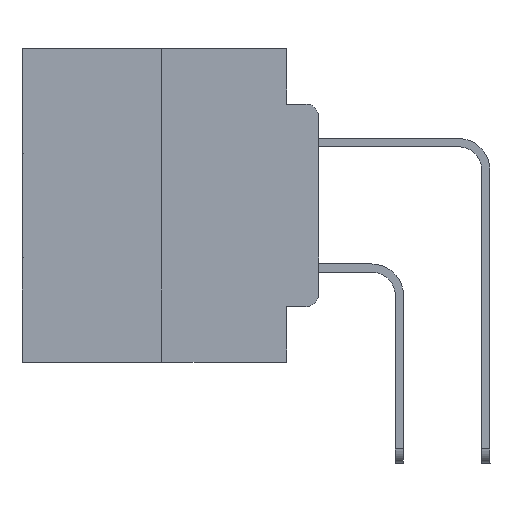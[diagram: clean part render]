
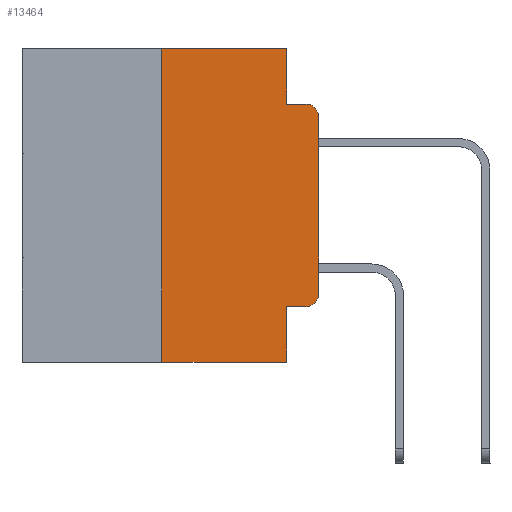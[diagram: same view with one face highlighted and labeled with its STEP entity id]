
A CAD part, left-side view. The second image highlights one B-rep face of the part: STEP entity #13464.
In plain terms, the highlighted planar face has unit normal (-1, 0, 0).
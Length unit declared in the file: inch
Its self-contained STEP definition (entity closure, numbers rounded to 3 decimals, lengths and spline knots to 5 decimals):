
#672 = LINE ( 'NONE', #13309, #23702 ) ;
#1261 = EDGE_CURVE ( 'NONE', #27705, #19291, #21496, .T. ) ;
#1399 = VERTEX_POINT ( 'NONE', #1431 ) ;
#1431 = CARTESIAN_POINT ( 'NONE',  ( 0., 0.25, 0. ) ) ;
#1716 = DIRECTION ( 'NONE',  ( 0., -1., 0. ) ) ;
#2072 = LINE ( 'NONE', #10075, #24971 ) ;
#3303 = CARTESIAN_POINT ( 'NONE',  ( 0., 0.051, -0.0885 ) ) ;
#3794 = ORIENTED_EDGE ( 'NONE', *, *, #26497, .F. ) ;
#3859 = VECTOR ( 'NONE', #27994, 39.37008 ) ;
#4047 = CARTESIAN_POINT ( 'NONE',  ( 0., 0.473, -0.5 ) ) ;
#4051 = AXIS2_PLACEMENT_3D ( 'NONE', #20321, #6572, #22577 ) ;
#4823 = VERTEX_POINT ( 'NONE', #15641 ) ;
#5180 = DIRECTION ( 'NONE',  ( 0., 0., 1. ) ) ;
#5366 = CARTESIAN_POINT ( 'NONE',  ( 0., 0.473, 0. ) ) ;
#5532 = DIRECTION ( 'NONE',  ( 0., 0., -1. ) ) ;
#6572 = DIRECTION ( 'NONE',  ( -1., 0., 0. ) ) ;
#7232 = ORIENTED_EDGE ( 'NONE', *, *, #22490, .T. ) ;
#7613 = ORIENTED_EDGE ( 'NONE', *, *, #24876, .T. ) ;
#7745 = ORIENTED_EDGE ( 'NONE', *, *, #11235, .F. ) ;
#7781 = VECTOR ( 'NONE', #28995, 39.37008 ) ;
#7864 = ORIENTED_EDGE ( 'NONE', *, *, #23756, .T. ) ;
#8063 = ORIENTED_EDGE ( 'NONE', *, *, #9125, .F. ) ;
#8181 = ORIENTED_EDGE ( 'NONE', *, *, #21394, .F. ) ;
#8349 = ORIENTED_EDGE ( 'NONE', *, *, #8543, .T. ) ;
#8543 = EDGE_CURVE ( 'NONE', #16999, #19291, #11043, .T. ) ;
#8806 = ORIENTED_EDGE ( 'NONE', *, *, #1261, .F. ) ;
#9125 = EDGE_CURVE ( 'NONE', #13517, #1399, #29331, .T. ) ;
#9257 = CARTESIAN_POINT ( 'NONE',  ( 0., 0., -0.1085 ) ) ;
#9340 = VECTOR ( 'NONE', #10320, 39.37008 ) ;
#9642 = VECTOR ( 'NONE', #5180, 39.37008 ) ;
#10075 = CARTESIAN_POINT ( 'NONE',  ( 0., 0.051, 0. ) ) ;
#10145 = CARTESIAN_POINT ( 'NONE',  ( 0., 0.051, -0.0885 ) ) ;
#10320 = DIRECTION ( 'NONE',  ( 0., -1., 0. ) ) ;
#10757 = LINE ( 'NONE', #5366, #3859 ) ;
#10809 = EDGE_LOOP ( 'NONE', ( #10975, #8349, #8806, #8181, #3794, #8063, #7864, #7745, #7613, #7232 ) ) ;
#10820 = CARTESIAN_POINT ( 'NONE',  ( 0., 0.02, -0.3915 ) ) ;
#10975 = ORIENTED_EDGE ( 'NONE', *, *, #15307, .T. ) ;
#11043 = CIRCLE ( 'NONE', #4051, 0.02 ) ;
#11235 = EDGE_CURVE ( 'NONE', #19425, #22166, #672, .T. ) ;
#11319 = VECTOR ( 'NONE', #1716, 39.37008 ) ;
#11891 = CARTESIAN_POINT ( 'NONE',  ( 0., 0.051, -0.4115 ) ) ;
#12069 = CARTESIAN_POINT ( 'NONE',  ( 0., 0., 0. ) ) ;
#12342 = AXIS2_PLACEMENT_3D ( 'NONE', #22597, #27020, #13566 ) ;
#13135 = DIRECTION ( 'NONE',  ( 0., 0., -1. ) ) ;
#13305 = CARTESIAN_POINT ( 'NONE',  ( 0., 0.051, -0.4115 ) ) ;
#13309 = CARTESIAN_POINT ( 'NONE',  ( 0., 0.051, 0. ) ) ;
#13464 = ADVANCED_FACE ( 'NONE', ( #18714 ), #29178, .F. ) ;
#13517 = VERTEX_POINT ( 'NONE', #22886 ) ;
#13566 = DIRECTION ( 'NONE',  ( 0., 0., -1. ) ) ;
#13632 = AXIS2_PLACEMENT_3D ( 'NONE', #10820, #26624, #13135 ) ;
#14188 = VERTEX_POINT ( 'NONE', #27700 ) ;
#15152 = CARTESIAN_POINT ( 'NONE',  ( 0., 0.25, 0. ) ) ;
#15307 = EDGE_CURVE ( 'NONE', #17213, #16999, #27666, .T. ) ;
#15641 = CARTESIAN_POINT ( 'NONE',  ( 0., 0.02, -0.4115 ) ) ;
#16999 = VERTEX_POINT ( 'NONE', #9257 ) ;
#17213 = VERTEX_POINT ( 'NONE', #23745 ) ;
#18714 = FACE_OUTER_BOUND ( 'NONE', #10809, .T. ) ;
#19291 = VERTEX_POINT ( 'NONE', #29048 ) ;
#19425 = VERTEX_POINT ( 'NONE', #11891 ) ;
#20321 = CARTESIAN_POINT ( 'NONE',  ( 0., 0.02, -0.1085 ) ) ;
#21130 = CARTESIAN_POINT ( 'NONE',  ( 0., 0.051, -0.5 ) ) ;
#21394 = EDGE_CURVE ( 'NONE', #14188, #27705, #2072, .T. ) ;
#21496 = LINE ( 'NONE', #3303, #9340 ) ;
#22166 = VERTEX_POINT ( 'NONE', #21130 ) ;
#22490 = EDGE_CURVE ( 'NONE', #4823, #17213, #25253, .T. ) ;
#22577 = DIRECTION ( 'NONE',  ( 0., 0., -1. ) ) ;
#22597 = CARTESIAN_POINT ( 'NONE',  ( 0., 0.473, 0. ) ) ;
#22886 = CARTESIAN_POINT ( 'NONE',  ( 0., 0.25, -0.5 ) ) ;
#23448 = VECTOR ( 'NONE', #24094, 39.37008 ) ;
#23702 = VECTOR ( 'NONE', #24557, 39.37008 ) ;
#23745 = CARTESIAN_POINT ( 'NONE',  ( 0., 0., -0.3915 ) ) ;
#23756 = EDGE_CURVE ( 'NONE', #13517, #22166, #25867, .T. ) ;
#24075 = LINE ( 'NONE', #13305, #11319 ) ;
#24094 = DIRECTION ( 'NONE',  ( 0., 0., 1. ) ) ;
#24557 = DIRECTION ( 'NONE',  ( 0., 0., -1. ) ) ;
#24876 = EDGE_CURVE ( 'NONE', #19425, #4823, #24075, .T. ) ;
#24971 = VECTOR ( 'NONE', #5532, 39.37008 ) ;
#25253 = CIRCLE ( 'NONE', #13632, 0.02 ) ;
#25867 = LINE ( 'NONE', #4047, #7781 ) ;
#26497 = EDGE_CURVE ( 'NONE', #1399, #14188, #10757, .T. ) ;
#26624 = DIRECTION ( 'NONE',  ( -1., 0., 0. ) ) ;
#27020 = DIRECTION ( 'NONE',  ( 1., 0., 0. ) ) ;
#27666 = LINE ( 'NONE', #12069, #9642 ) ;
#27700 = CARTESIAN_POINT ( 'NONE',  ( 0., 0.051, 0. ) ) ;
#27705 = VERTEX_POINT ( 'NONE', #10145 ) ;
#27994 = DIRECTION ( 'NONE',  ( 0., -1., 0. ) ) ;
#28995 = DIRECTION ( 'NONE',  ( 0., -1., 0. ) ) ;
#29048 = CARTESIAN_POINT ( 'NONE',  ( 0., 0.02, -0.0885 ) ) ;
#29178 = PLANE ( 'NONE',  #12342 ) ;
#29331 = LINE ( 'NONE', #15152, #23448 ) ;
